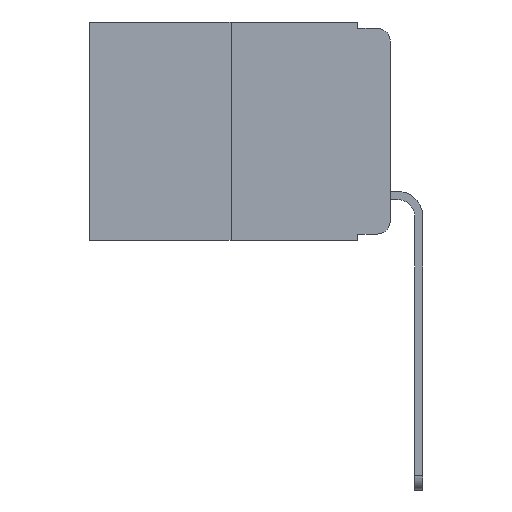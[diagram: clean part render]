
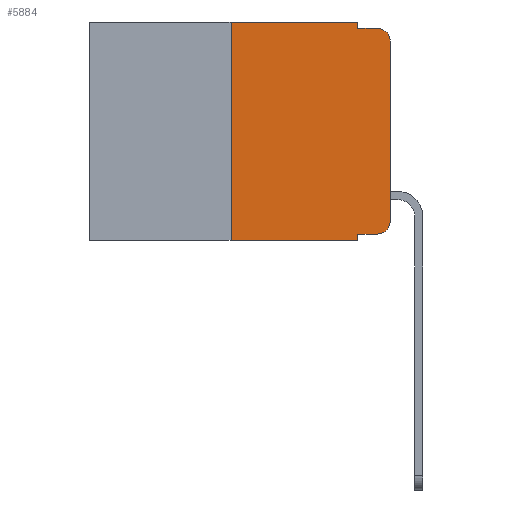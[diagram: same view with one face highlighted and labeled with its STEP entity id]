
A CAD part, left-side view. The second image highlights one B-rep face of the part: STEP entity #5884.
In plain terms, the highlighted planar face has unit normal (-1, 0, 0).
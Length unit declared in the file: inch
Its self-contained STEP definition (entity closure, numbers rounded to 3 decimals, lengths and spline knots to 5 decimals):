
#58 = ORIENTED_EDGE ( 'NONE', *, *, #3029, .F. ) ;
#133 = VERTEX_POINT ( 'NONE', #15973 ) ;
#1190 = VERTEX_POINT ( 'NONE', #15927 ) ;
#1356 = EDGE_CURVE ( 'NONE', #2606, #8438, #6259, .T. ) ;
#1697 = DIRECTION ( 'NONE',  ( -1., 0., 0. ) ) ;
#1908 = DIRECTION ( 'NONE',  ( -1., 0., 0. ) ) ;
#1920 = CARTESIAN_POINT ( 'NONE',  ( 0., 0.051, 0. ) ) ;
#2149 = CARTESIAN_POINT ( 'NONE',  ( 0., 0.051, 0. ) ) ;
#2260 = VECTOR ( 'NONE', #4010, 39.37008 ) ;
#2448 = DIRECTION ( 'NONE',  ( 0., -1., 0. ) ) ;
#2606 = VERTEX_POINT ( 'NONE', #14760 ) ;
#2746 = CARTESIAN_POINT ( 'NONE',  ( 0., 0.051, -0.01 ) ) ;
#3029 = EDGE_CURVE ( 'NONE', #14293, #14167, #3774, .T. ) ;
#3152 = DIRECTION ( 'NONE',  ( 0., 0., 1. ) ) ;
#3216 = DIRECTION ( 'NONE',  ( 0., -1., 0. ) ) ;
#3266 = EDGE_CURVE ( 'NONE', #11494, #4549, #6596, .T. ) ;
#3549 = CARTESIAN_POINT ( 'NONE',  ( 0., 0.473, 0. ) ) ;
#3602 = PLANE ( 'NONE',  #3912 ) ;
#3774 = LINE ( 'NONE', #12950, #16511 ) ;
#3912 = AXIS2_PLACEMENT_3D ( 'NONE', #3549, #12622, #4920 ) ;
#4010 = DIRECTION ( 'NONE',  ( 0., -1., 0. ) ) ;
#4258 = EDGE_CURVE ( 'NONE', #14293, #133, #10365, .T. ) ;
#4485 = VECTOR ( 'NONE', #9074, 39.37008 ) ;
#4546 = ORIENTED_EDGE ( 'NONE', *, *, #4258, .T. ) ;
#4549 = VERTEX_POINT ( 'NONE', #15661 ) ;
#4570 = VECTOR ( 'NONE', #3216, 39.37008 ) ;
#4920 = DIRECTION ( 'NONE',  ( 0., 0., -1. ) ) ;
#4958 = ORIENTED_EDGE ( 'NONE', *, *, #5471, .T. ) ;
#5404 = CARTESIAN_POINT ( 'NONE',  ( 0., 0., 0. ) ) ;
#5471 = EDGE_CURVE ( 'NONE', #133, #8211, #7100, .T. ) ;
#5633 = CARTESIAN_POINT ( 'NONE',  ( 0., 0.25, -0.343 ) ) ;
#5884 = ADVANCED_FACE ( 'NONE', ( #14305 ), #3602, .F. ) ;
#6259 = LINE ( 'NONE', #16299, #15977 ) ;
#6268 = LINE ( 'NONE', #1920, #13098 ) ;
#6596 = CIRCLE ( 'NONE', #10783, 0.02 ) ;
#6803 = CARTESIAN_POINT ( 'NONE',  ( 0., 0., -0.03 ) ) ;
#6917 = ORIENTED_EDGE ( 'NONE', *, *, #1356, .F. ) ;
#6925 = VECTOR ( 'NONE', #2448, 39.37008 ) ;
#7074 = EDGE_LOOP ( 'NONE', ( #12376, #16064, #10147, #11395, #6917, #12002, #12789, #58, #4546, #4958 ) ) ;
#7100 = CIRCLE ( 'NONE', #13174, 0.02 ) ;
#8211 = VERTEX_POINT ( 'NONE', #12045 ) ;
#8344 = CARTESIAN_POINT ( 'NONE',  ( 0., 0.473, -0.343 ) ) ;
#8438 = VERTEX_POINT ( 'NONE', #2149 ) ;
#8663 = DIRECTION ( 'NONE',  ( 0., -1., 0. ) ) ;
#8701 = VECTOR ( 'NONE', #3152, 39.37008 ) ;
#8759 = LINE ( 'NONE', #2746, #2260 ) ;
#9074 = DIRECTION ( 'NONE',  ( 0., 0., 1. ) ) ;
#9495 = CARTESIAN_POINT ( 'NONE',  ( 0., 0.02, -0.03 ) ) ;
#9701 = CARTESIAN_POINT ( 'NONE',  ( 0., 0.02, -0.313 ) ) ;
#10147 = ORIENTED_EDGE ( 'NONE', *, *, #11396, .F. ) ;
#10200 = CARTESIAN_POINT ( 'NONE',  ( 0., 0.051, -0.333 ) ) ;
#10326 = VERTEX_POINT ( 'NONE', #5633 ) ;
#10365 = LINE ( 'NONE', #10200, #6925 ) ;
#10697 = EDGE_CURVE ( 'NONE', #10326, #14167, #11431, .T. ) ;
#10783 = AXIS2_PLACEMENT_3D ( 'NONE', #9495, #1697, #10789 ) ;
#10789 = DIRECTION ( 'NONE',  ( 0., 0., -1. ) ) ;
#10925 = LINE ( 'NONE', #15419, #4485 ) ;
#11011 = DIRECTION ( 'NONE',  ( 0., 0., -1. ) ) ;
#11395 = ORIENTED_EDGE ( 'NONE', *, *, #15874, .F. ) ;
#11396 = EDGE_CURVE ( 'NONE', #1190, #4549, #8759, .T. ) ;
#11431 = LINE ( 'NONE', #8344, #4570 ) ;
#11494 = VERTEX_POINT ( 'NONE', #6803 ) ;
#12002 = ORIENTED_EDGE ( 'NONE', *, *, #15067, .F. ) ;
#12045 = CARTESIAN_POINT ( 'NONE',  ( 0., 0., -0.313 ) ) ;
#12376 = ORIENTED_EDGE ( 'NONE', *, *, #13600, .T. ) ;
#12447 = DIRECTION ( 'NONE',  ( 0., 0., -1. ) ) ;
#12622 = DIRECTION ( 'NONE',  ( 1., 0., 0. ) ) ;
#12789 = ORIENTED_EDGE ( 'NONE', *, *, #10697, .T. ) ;
#12950 = CARTESIAN_POINT ( 'NONE',  ( 0., 0.051, 0. ) ) ;
#13098 = VECTOR ( 'NONE', #12447, 39.37008 ) ;
#13108 = CARTESIAN_POINT ( 'NONE',  ( 0., 0.051, -0.343 ) ) ;
#13174 = AXIS2_PLACEMENT_3D ( 'NONE', #9701, #1908, #11011 ) ;
#13600 = EDGE_CURVE ( 'NONE', #8211, #11494, #15485, .T. ) ;
#14167 = VERTEX_POINT ( 'NONE', #13108 ) ;
#14193 = DIRECTION ( 'NONE',  ( 0., 0., -1. ) ) ;
#14293 = VERTEX_POINT ( 'NONE', #16176 ) ;
#14305 = FACE_OUTER_BOUND ( 'NONE', #7074, .T. ) ;
#14760 = CARTESIAN_POINT ( 'NONE',  ( 0., 0.25, 0. ) ) ;
#15067 = EDGE_CURVE ( 'NONE', #10326, #2606, #10925, .T. ) ;
#15419 = CARTESIAN_POINT ( 'NONE',  ( 0., 0.25, 0. ) ) ;
#15485 = LINE ( 'NONE', #5404, #8701 ) ;
#15661 = CARTESIAN_POINT ( 'NONE',  ( 0., 0.02, -0.01 ) ) ;
#15874 = EDGE_CURVE ( 'NONE', #8438, #1190, #6268, .T. ) ;
#15927 = CARTESIAN_POINT ( 'NONE',  ( 0., 0.051, -0.01 ) ) ;
#15973 = CARTESIAN_POINT ( 'NONE',  ( 0., 0.02, -0.333 ) ) ;
#15977 = VECTOR ( 'NONE', #8663, 39.37008 ) ;
#16064 = ORIENTED_EDGE ( 'NONE', *, *, #3266, .T. ) ;
#16176 = CARTESIAN_POINT ( 'NONE',  ( 0., 0.051, -0.333 ) ) ;
#16299 = CARTESIAN_POINT ( 'NONE',  ( 0., 0.473, 0. ) ) ;
#16511 = VECTOR ( 'NONE', #14193, 39.37008 ) ;
